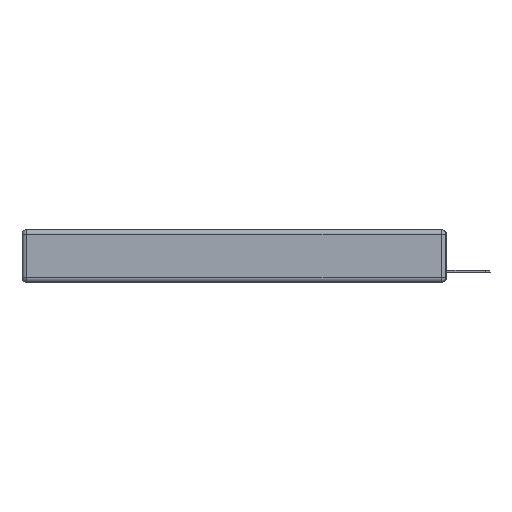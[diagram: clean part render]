
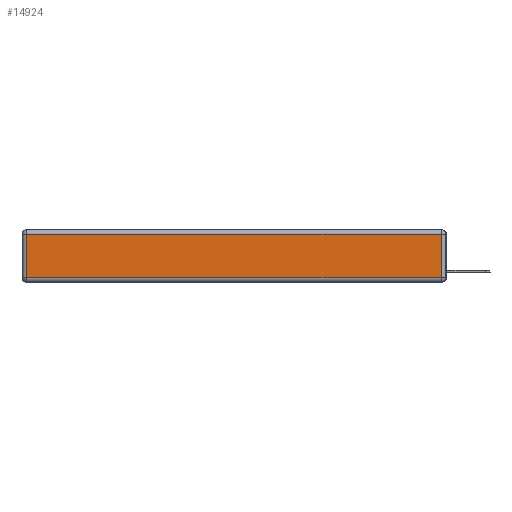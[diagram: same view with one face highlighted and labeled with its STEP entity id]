
A CAD part, left-side view. The second image highlights one B-rep face of the part: STEP entity #14924.
In plain terms, the highlighted planar face has unit normal (-1, 0, 0).
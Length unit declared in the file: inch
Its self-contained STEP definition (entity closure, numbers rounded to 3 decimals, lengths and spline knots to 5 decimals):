
#493 = EDGE_CURVE ( 'NONE', #1763, #9848, #6563, .T. ) ;
#864 = VECTOR ( 'NONE', #3955, 39.37008 ) ;
#1036 = CARTESIAN_POINT ( 'NONE',  ( 0., 0.03, -0.343 ) ) ;
#1763 = VERTEX_POINT ( 'NONE', #7221 ) ;
#2207 = CARTESIAN_POINT ( 'NONE',  ( 0., 2.72, -0.03 ) ) ;
#2382 = PLANE ( 'NONE',  #4297 ) ;
#2621 = DIRECTION ( 'NONE',  ( 0., 1., 0. ) ) ;
#2748 = LINE ( 'NONE', #4787, #7997 ) ;
#3204 = DIRECTION ( 'NONE',  ( 0., -1., 0. ) ) ;
#3418 = CARTESIAN_POINT ( 'NONE',  ( 0., 0., -0.313 ) ) ;
#3462 = FACE_OUTER_BOUND ( 'NONE', #10383, .T. ) ;
#3955 = DIRECTION ( 'NONE',  ( 0., 0., 1. ) ) ;
#4297 = AXIS2_PLACEMENT_3D ( 'NONE', #7591, #12524, #8761 ) ;
#4320 = ORIENTED_EDGE ( 'NONE', *, *, #6544, .T. ) ;
#4787 = CARTESIAN_POINT ( 'NONE',  ( 0., 2.72, -0.343 ) ) ;
#4917 = VERTEX_POINT ( 'NONE', #7622 ) ;
#5677 = LINE ( 'NONE', #3418, #7099 ) ;
#6143 = ORIENTED_EDGE ( 'NONE', *, *, #7823, .T. ) ;
#6544 = EDGE_CURVE ( 'NONE', #9848, #4917, #2748, .T. ) ;
#6563 = LINE ( 'NONE', #10354, #10412 ) ;
#7099 = VECTOR ( 'NONE', #3204, 39.37008 ) ;
#7221 = CARTESIAN_POINT ( 'NONE',  ( 0., 0.03, -0.03 ) ) ;
#7591 = CARTESIAN_POINT ( 'NONE',  ( 0., 0., -0.343 ) ) ;
#7622 = CARTESIAN_POINT ( 'NONE',  ( 0., 2.72, -0.313 ) ) ;
#7823 = EDGE_CURVE ( 'NONE', #12263, #1763, #8131, .T. ) ;
#7997 = VECTOR ( 'NONE', #12599, 39.37008 ) ;
#8131 = LINE ( 'NONE', #1036, #864 ) ;
#8761 = DIRECTION ( 'NONE',  ( 0., 0., 1. ) ) ;
#8967 = ORIENTED_EDGE ( 'NONE', *, *, #14833, .T. ) ;
#9848 = VERTEX_POINT ( 'NONE', #2207 ) ;
#10354 = CARTESIAN_POINT ( 'NONE',  ( 0., 2.75, -0.03 ) ) ;
#10383 = EDGE_LOOP ( 'NONE', ( #8967, #6143, #11178, #4320 ) ) ;
#10412 = VECTOR ( 'NONE', #2621, 39.37008 ) ;
#11178 = ORIENTED_EDGE ( 'NONE', *, *, #493, .T. ) ;
#12263 = VERTEX_POINT ( 'NONE', #14855 ) ;
#12524 = DIRECTION ( 'NONE',  ( -1., 0., 0. ) ) ;
#12599 = DIRECTION ( 'NONE',  ( 0., 0., -1. ) ) ;
#14833 = EDGE_CURVE ( 'NONE', #4917, #12263, #5677, .T. ) ;
#14855 = CARTESIAN_POINT ( 'NONE',  ( 0., 0.03, -0.313 ) ) ;
#14924 = ADVANCED_FACE ( 'NONE', ( #3462 ), #2382, .T. ) ;
